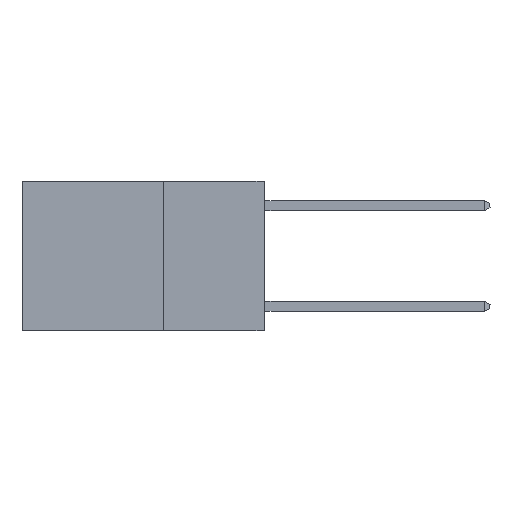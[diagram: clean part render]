
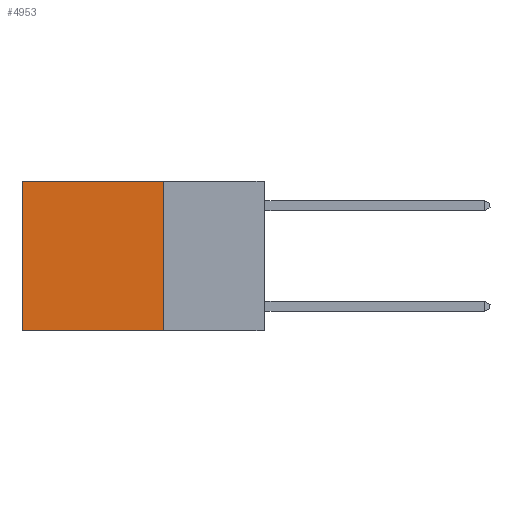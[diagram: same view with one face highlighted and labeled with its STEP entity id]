
A CAD part, left-side view. The second image highlights one B-rep face of the part: STEP entity #4953.
In plain terms, the highlighted planar face has unit normal (-1, 0, 0).
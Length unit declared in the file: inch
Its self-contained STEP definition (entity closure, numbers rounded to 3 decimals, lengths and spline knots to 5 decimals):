
#164 = EDGE_LOOP ( 'NONE', ( #5760, #1039, #7403, #3651 ) ) ;
#185 = FACE_OUTER_BOUND ( 'NONE', #164, .T. ) ;
#354 = LINE ( 'NONE', #521, #10077 ) ;
#521 = CARTESIAN_POINT ( 'NONE',  ( 0.2625, 0.25, 0. ) ) ;
#1039 = ORIENTED_EDGE ( 'NONE', *, *, #11159, .F. ) ;
#1517 = CARTESIAN_POINT ( 'NONE',  ( 0.2625, 0.6, 0. ) ) ;
#1572 = VERTEX_POINT ( 'NONE', #12515 ) ;
#2705 = VECTOR ( 'NONE', #8439, 39.37008 ) ;
#2976 = VERTEX_POINT ( 'NONE', #10977 ) ;
#3651 = ORIENTED_EDGE ( 'NONE', *, *, #8252, .T. ) ;
#4140 = VERTEX_POINT ( 'NONE', #10312 ) ;
#4239 = VECTOR ( 'NONE', #6349, 39.37008 ) ;
#4908 = VECTOR ( 'NONE', #7944, 39.37008 ) ;
#4953 = ADVANCED_FACE ( 'NONE', ( #185 ), #11751, .F. ) ;
#5445 = CARTESIAN_POINT ( 'NONE',  ( 0.2625, 0.25, -0.37 ) ) ;
#5760 = ORIENTED_EDGE ( 'NONE', *, *, #6047, .T. ) ;
#6047 = EDGE_CURVE ( 'NONE', #7964, #2976, #12307, .T. ) ;
#6153 = CARTESIAN_POINT ( 'NONE',  ( 0.2625, 0.25, 0. ) ) ;
#6174 = AXIS2_PLACEMENT_3D ( 'NONE', #6153, #7155, #12219 ) ;
#6347 = DIRECTION ( 'NONE',  ( 0., 0., -1. ) ) ;
#6349 = DIRECTION ( 'NONE',  ( 0., 1., 0. ) ) ;
#7155 = DIRECTION ( 'NONE',  ( 1., 0., 0. ) ) ;
#7403 = ORIENTED_EDGE ( 'NONE', *, *, #10027, .F. ) ;
#7944 = DIRECTION ( 'NONE',  ( 0., 1., 0. ) ) ;
#7964 = VERTEX_POINT ( 'NONE', #8047 ) ;
#8047 = CARTESIAN_POINT ( 'NONE',  ( 0.2625, 0.6, 0. ) ) ;
#8252 = EDGE_CURVE ( 'NONE', #1572, #7964, #8591, .T. ) ;
#8439 = DIRECTION ( 'NONE',  ( 0., 0., -1. ) ) ;
#8591 = LINE ( 'NONE', #9862, #4908 ) ;
#9862 = CARTESIAN_POINT ( 'NONE',  ( 0.2625, 0.25, 0. ) ) ;
#10027 = EDGE_CURVE ( 'NONE', #1572, #4140, #354, .T. ) ;
#10077 = VECTOR ( 'NONE', #6347, 39.37008 ) ;
#10312 = CARTESIAN_POINT ( 'NONE',  ( 0.2625, 0.25, -0.37 ) ) ;
#10977 = CARTESIAN_POINT ( 'NONE',  ( 0.2625, 0.6, -0.37 ) ) ;
#11159 = EDGE_CURVE ( 'NONE', #4140, #2976, #12188, .T. ) ;
#11751 = PLANE ( 'NONE',  #6174 ) ;
#12188 = LINE ( 'NONE', #5445, #4239 ) ;
#12219 = DIRECTION ( 'NONE',  ( 0., 0., -1. ) ) ;
#12307 = LINE ( 'NONE', #1517, #2705 ) ;
#12515 = CARTESIAN_POINT ( 'NONE',  ( 0.2625, 0.25, 0. ) ) ;
